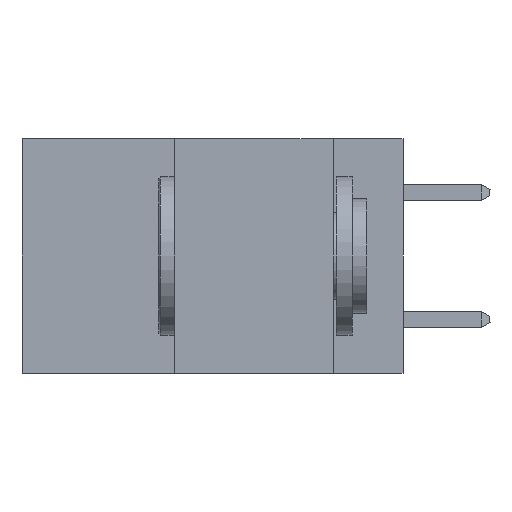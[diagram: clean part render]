
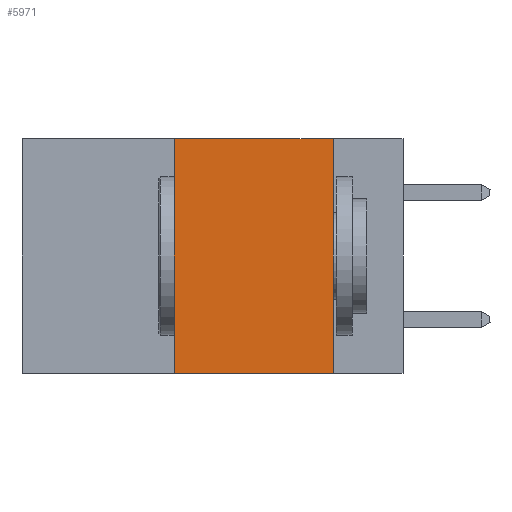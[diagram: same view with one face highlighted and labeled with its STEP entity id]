
A CAD part, left-side view. The second image highlights one B-rep face of the part: STEP entity #5971.
In plain terms, the highlighted planar face has unit normal (-1, 0, 0).
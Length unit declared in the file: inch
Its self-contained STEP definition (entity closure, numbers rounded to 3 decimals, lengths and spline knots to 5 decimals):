
#1479 = DIRECTION ( 'NONE',  ( 0., 0., -1. ) ) ;
#2573 = FACE_OUTER_BOUND ( 'NONE', #6621, .T. ) ;
#2789 = CARTESIAN_POINT ( 'NONE',  ( 0., 0.11, 0. ) ) ;
#3523 = VERTEX_POINT ( 'NONE', #31610 ) ;
#4115 = PLANE ( 'NONE',  #30656 ) ;
#5971 = ADVANCED_FACE ( 'NONE', ( #2573 ), #4115, .F. ) ;
#6621 = EDGE_LOOP ( 'NONE', ( #17993, #20453, #37639, #23374 ) ) ;
#7230 = DIRECTION ( 'NONE',  ( 0., 0., 1. ) ) ;
#7364 = VECTOR ( 'NONE', #35730, 39.37008 ) ;
#11241 = DIRECTION ( 'NONE',  ( 0., -1., 0. ) ) ;
#12744 = CARTESIAN_POINT ( 'NONE',  ( 0., 0.6, 0. ) ) ;
#13447 = DIRECTION ( 'NONE',  ( 0., 0., -1. ) ) ;
#13500 = CARTESIAN_POINT ( 'NONE',  ( 0., 0.36, -0.37 ) ) ;
#14452 = EDGE_CURVE ( 'NONE', #21647, #17714, #17012, .T. ) ;
#14566 = EDGE_CURVE ( 'NONE', #21905, #17714, #17903, .T. ) ;
#15415 = CARTESIAN_POINT ( 'NONE',  ( 0., 0.6, -0.37 ) ) ;
#16842 = VECTOR ( 'NONE', #11241, 39.37008 ) ;
#17012 = LINE ( 'NONE', #15415, #7364 ) ;
#17207 = LINE ( 'NONE', #21294, #33554 ) ;
#17714 = VERTEX_POINT ( 'NONE', #25046 ) ;
#17903 = LINE ( 'NONE', #33313, #30643 ) ;
#17993 = ORIENTED_EDGE ( 'NONE', *, *, #14566, .F. ) ;
#18336 = DIRECTION ( 'NONE',  ( 1., 0., 0. ) ) ;
#20308 = CARTESIAN_POINT ( 'NONE',  ( 0., 0.6, 0. ) ) ;
#20453 = ORIENTED_EDGE ( 'NONE', *, *, #36136, .F. ) ;
#21294 = CARTESIAN_POINT ( 'NONE',  ( 0., 0.36, 0. ) ) ;
#21647 = VERTEX_POINT ( 'NONE', #13500 ) ;
#21905 = VERTEX_POINT ( 'NONE', #2789 ) ;
#23374 = ORIENTED_EDGE ( 'NONE', *, *, #14452, .T. ) ;
#24562 = LINE ( 'NONE', #20308, #16842 ) ;
#25046 = CARTESIAN_POINT ( 'NONE',  ( 0., 0.11, -0.37 ) ) ;
#30643 = VECTOR ( 'NONE', #13447, 39.37008 ) ;
#30656 = AXIS2_PLACEMENT_3D ( 'NONE', #12744, #18336, #1479 ) ;
#31610 = CARTESIAN_POINT ( 'NONE',  ( 0., 0.36, 0. ) ) ;
#33313 = CARTESIAN_POINT ( 'NONE',  ( 0., 0.11, 0. ) ) ;
#33554 = VECTOR ( 'NONE', #7230, 39.37008 ) ;
#35730 = DIRECTION ( 'NONE',  ( 0., -1., 0. ) ) ;
#36136 = EDGE_CURVE ( 'NONE', #3523, #21905, #24562, .T. ) ;
#37468 = EDGE_CURVE ( 'NONE', #21647, #3523, #17207, .T. ) ;
#37639 = ORIENTED_EDGE ( 'NONE', *, *, #37468, .F. ) ;
